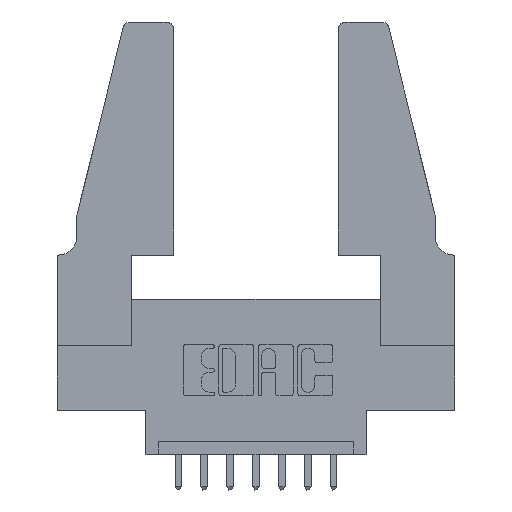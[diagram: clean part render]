
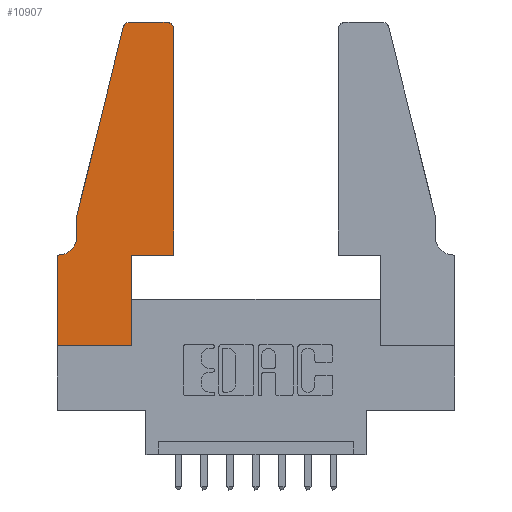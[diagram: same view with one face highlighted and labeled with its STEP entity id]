
A CAD part, top view. The second image highlights one B-rep face of the part: STEP entity #10907.
In plain terms, the highlighted planar face has unit normal (0, 0, 1).
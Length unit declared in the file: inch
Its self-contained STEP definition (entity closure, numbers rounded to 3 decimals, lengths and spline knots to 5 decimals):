
#19 = CARTESIAN_POINT ( 'NONE',  ( 0.284, 1.22, 0.37 ) ) ;
#197 = DIRECTION ( 'NONE',  ( 0., -1., 0. ) ) ;
#254 = CARTESIAN_POINT ( 'NONE',  ( 0.4505, 1.22, 0.37 ) ) ;
#389 = DIRECTION ( 'NONE',  ( 0., 1., 0. ) ) ;
#526 = VECTOR ( 'NONE', #3618, 39.37008 ) ;
#636 = CARTESIAN_POINT ( 'NONE',  ( 0.2605, 1.25, 0.37 ) ) ;
#781 = DIRECTION ( 'NONE',  ( -0.239, -0.971, 0. ) ) ;
#833 = CARTESIAN_POINT ( 'NONE',  ( 0.0755, 0.5, 0.37 ) ) ;
#901 = PLANE ( 'NONE',  #5251 ) ;
#1079 = DIRECTION ( 'NONE',  ( 0., 1., 0. ) ) ;
#1259 = VECTOR ( 'NONE', #10516, 39.37008 ) ;
#1412 = EDGE_CURVE ( 'NONE', #7681, #4848, #2470, .T. ) ;
#1493 = DIRECTION ( 'NONE',  ( 1., 0., 0. ) ) ;
#1522 = AXIS2_PLACEMENT_3D ( 'NONE', #9233, #10176, #10297 ) ;
#1580 = CIRCLE ( 'NONE', #4860, 0.07 ) ;
#1715 = LINE ( 'NONE', #7816, #11687 ) ;
#1811 = CARTESIAN_POINT ( 'NONE',  ( 0., 0.35, 0.37 ) ) ;
#2047 = VECTOR ( 'NONE', #389, 39.37008 ) ;
#2191 = EDGE_CURVE ( 'NONE', #3181, #9381, #1580, .T. ) ;
#2324 = CARTESIAN_POINT ( 'NONE',  ( 0., 0.35, 0.37 ) ) ;
#2440 = CARTESIAN_POINT ( 'NONE',  ( 0., 0., 0.37 ) ) ;
#2470 = LINE ( 'NONE', #3655, #9068 ) ;
#2678 = DIRECTION ( 'NONE',  ( 0., 0., 1. ) ) ;
#2781 = DIRECTION ( 'NONE',  ( 1., 0., 0. ) ) ;
#2865 = CIRCLE ( 'NONE', #6465, 0.03 ) ;
#3181 = VERTEX_POINT ( 'NONE', #9311 ) ;
#3301 = DIRECTION ( 'NONE',  ( 0., 0., -1. ) ) ;
#3359 = LINE ( 'NONE', #6057, #2047 ) ;
#3409 = FACE_OUTER_BOUND ( 'NONE', #5516, .T. ) ;
#3443 = ORIENTED_EDGE ( 'NONE', *, *, #10785, .T. ) ;
#3618 = DIRECTION ( 'NONE',  ( 0., -1., 0. ) ) ;
#3644 = ORIENTED_EDGE ( 'NONE', *, *, #8341, .T. ) ;
#3655 = CARTESIAN_POINT ( 'NONE',  ( 0.0755, 0.5, 0.37 ) ) ;
#3844 = EDGE_CURVE ( 'NONE', #6842, #7681, #2865, .T. ) ;
#3874 = LINE ( 'NONE', #2440, #11649 ) ;
#3944 = VECTOR ( 'NONE', #12139, 39.37008 ) ;
#4125 = ORIENTED_EDGE ( 'NONE', *, *, #5172, .T. ) ;
#4192 = ORIENTED_EDGE ( 'NONE', *, *, #3844, .T. ) ;
#4193 = VERTEX_POINT ( 'NONE', #9263 ) ;
#4224 = CARTESIAN_POINT ( 'NONE',  ( 0.25487, 1.22718, 0.37 ) ) ;
#4634 = DIRECTION ( 'NONE',  ( 1., 0., 0. ) ) ;
#4671 = LINE ( 'NONE', #9494, #1259 ) ;
#4693 = EDGE_CURVE ( 'NONE', #6059, #6842, #9378, .T. ) ;
#4779 = VERTEX_POINT ( 'NONE', #10986 ) ;
#4848 = VERTEX_POINT ( 'NONE', #833 ) ;
#4860 = AXIS2_PLACEMENT_3D ( 'NONE', #5108, #3301, #8156 ) ;
#5056 = CIRCLE ( 'NONE', #1522, 0.03 ) ;
#5108 = CARTESIAN_POINT ( 'NONE',  ( 0.0055, 0.42, 0.37 ) ) ;
#5131 = CARTESIAN_POINT ( 'NONE',  ( 0.0755, 0.5, 0.37 ) ) ;
#5172 = EDGE_CURVE ( 'NONE', #6151, #4193, #3359, .T. ) ;
#5251 = AXIS2_PLACEMENT_3D ( 'NONE', #1811, #2678, #4634 ) ;
#5516 = EDGE_LOOP ( 'NONE', ( #11246, #4192, #7954, #10458, #10792, #3443, #9989, #3644, #4125, #11016, #8777, #8488 ) ) ;
#5543 = CARTESIAN_POINT ( 'NONE',  ( 0.2865, 0., 0.37 ) ) ;
#6057 = CARTESIAN_POINT ( 'NONE',  ( 0.2865, 0.35, 0.37 ) ) ;
#6059 = VERTEX_POINT ( 'NONE', #9323 ) ;
#6151 = VERTEX_POINT ( 'NONE', #5543 ) ;
#6276 = VERTEX_POINT ( 'NONE', #254 ) ;
#6284 = DIRECTION ( 'NONE',  ( -1., 0., 0. ) ) ;
#6465 = AXIS2_PLACEMENT_3D ( 'NONE', #19, #9558, #2781 ) ;
#6666 = VECTOR ( 'NONE', #6284, 39.37008 ) ;
#6728 = EDGE_CURVE ( 'NONE', #11244, #4779, #10218, .T. ) ;
#6842 = VERTEX_POINT ( 'NONE', #6847 ) ;
#6847 = CARTESIAN_POINT ( 'NONE',  ( 0.284, 1.25, 0.37 ) ) ;
#6953 = EDGE_CURVE ( 'NONE', #8836, #6276, #1715, .T. ) ;
#7385 = EDGE_CURVE ( 'NONE', #4193, #8836, #4671, .T. ) ;
#7681 = VERTEX_POINT ( 'NONE', #4224 ) ;
#7816 = CARTESIAN_POINT ( 'NONE',  ( 0.4505, 0.35, 0.37 ) ) ;
#7954 = ORIENTED_EDGE ( 'NONE', *, *, #1412, .T. ) ;
#8156 = DIRECTION ( 'NONE',  ( -1., 0., 0. ) ) ;
#8227 = VECTOR ( 'NONE', #197, 39.37008 ) ;
#8341 = EDGE_CURVE ( 'NONE', #4779, #6151, #3874, .T. ) ;
#8488 = ORIENTED_EDGE ( 'NONE', *, *, #11393, .T. ) ;
#8639 = LINE ( 'NONE', #11011, #6666 ) ;
#8777 = ORIENTED_EDGE ( 'NONE', *, *, #6953, .T. ) ;
#8836 = VERTEX_POINT ( 'NONE', #9976 ) ;
#9068 = VECTOR ( 'NONE', #781, 39.37008 ) ;
#9233 = CARTESIAN_POINT ( 'NONE',  ( 0.4205, 1.22, 0.37 ) ) ;
#9263 = CARTESIAN_POINT ( 'NONE',  ( 0.2865, 0.35, 0.37 ) ) ;
#9311 = CARTESIAN_POINT ( 'NONE',  ( 0.0755, 0.42, 0.37 ) ) ;
#9323 = CARTESIAN_POINT ( 'NONE',  ( 0.4205, 1.25, 0.37 ) ) ;
#9378 = LINE ( 'NONE', #636, #3944 ) ;
#9381 = VERTEX_POINT ( 'NONE', #11633 ) ;
#9494 = CARTESIAN_POINT ( 'NONE',  ( 0.4505, 0.35, 0.37 ) ) ;
#9540 = CARTESIAN_POINT ( 'NONE',  ( 0., 0., 0.37 ) ) ;
#9558 = DIRECTION ( 'NONE',  ( 0., 0., 1. ) ) ;
#9976 = CARTESIAN_POINT ( 'NONE',  ( 0.4505, 0.35, 0.37 ) ) ;
#9989 = ORIENTED_EDGE ( 'NONE', *, *, #6728, .T. ) ;
#10176 = DIRECTION ( 'NONE',  ( 0., 0., 1. ) ) ;
#10218 = LINE ( 'NONE', #9540, #526 ) ;
#10297 = DIRECTION ( 'NONE',  ( 1., 0., 0. ) ) ;
#10458 = ORIENTED_EDGE ( 'NONE', *, *, #11220, .T. ) ;
#10516 = DIRECTION ( 'NONE',  ( 1., 0., 0. ) ) ;
#10785 = EDGE_CURVE ( 'NONE', #9381, #11244, #8639, .T. ) ;
#10792 = ORIENTED_EDGE ( 'NONE', *, *, #2191, .T. ) ;
#10907 = ADVANCED_FACE ( 'NONE', ( #3409 ), #901, .T. ) ;
#10986 = CARTESIAN_POINT ( 'NONE',  ( 0., 0., 0.37 ) ) ;
#11011 = CARTESIAN_POINT ( 'NONE',  ( 0.0755, 0.35, 0.37 ) ) ;
#11016 = ORIENTED_EDGE ( 'NONE', *, *, #7385, .T. ) ;
#11220 = EDGE_CURVE ( 'NONE', #4848, #3181, #11356, .T. ) ;
#11244 = VERTEX_POINT ( 'NONE', #2324 ) ;
#11246 = ORIENTED_EDGE ( 'NONE', *, *, #4693, .T. ) ;
#11356 = LINE ( 'NONE', #5131, #8227 ) ;
#11393 = EDGE_CURVE ( 'NONE', #6276, #6059, #5056, .T. ) ;
#11633 = CARTESIAN_POINT ( 'NONE',  ( 0.0055, 0.35, 0.37 ) ) ;
#11649 = VECTOR ( 'NONE', #1493, 39.37008 ) ;
#11687 = VECTOR ( 'NONE', #1079, 39.37008 ) ;
#12139 = DIRECTION ( 'NONE',  ( -1., 0., 0. ) ) ;
